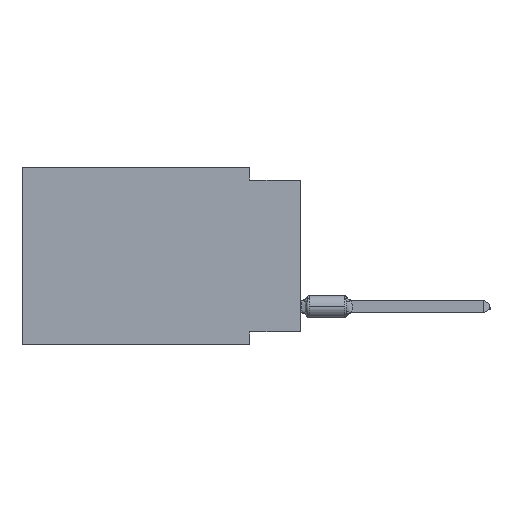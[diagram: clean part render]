
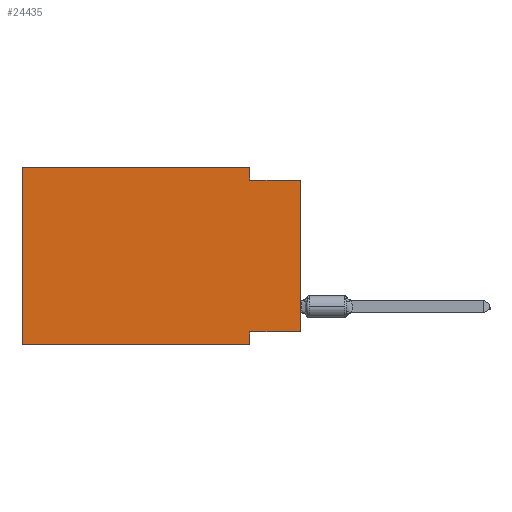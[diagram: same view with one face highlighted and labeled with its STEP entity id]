
A CAD part, left-side view. The second image highlights one B-rep face of the part: STEP entity #24435.
In plain terms, the highlighted planar face has unit normal (-1, 0, 0).
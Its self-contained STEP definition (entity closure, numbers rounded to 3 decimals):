
#930 = VECTOR ( 'NONE', #31908, 1000. ) ;
#1468 = ORIENTED_EDGE ( 'NONE', *, *, #15629, .T. ) ;
#1603 = VERTEX_POINT ( 'NONE', #9356 ) ;
#1657 = LINE ( 'NONE', #26154, #13521 ) ;
#1688 = LINE ( 'NONE', #13931, #12586 ) ;
#4065 = EDGE_CURVE ( 'NONE', #1603, #14126, #7188, .T. ) ;
#5180 = VECTOR ( 'NONE', #22248, 1000. ) ;
#5449 = AXIS2_PLACEMENT_3D ( 'NONE', #14521, #35636, #17737 ) ;
#5490 = ORIENTED_EDGE ( 'NONE', *, *, #20607, .F. ) ;
#6143 = DIRECTION ( 'NONE',  ( 0., -1., 0. ) ) ;
#7188 = LINE ( 'NONE', #19037, #5180 ) ;
#7659 = EDGE_CURVE ( 'NONE', #29925, #8269, #30034, .T. ) ;
#7812 = LINE ( 'NONE', #26083, #930 ) ;
#8269 = VERTEX_POINT ( 'NONE', #36052 ) ;
#8613 = EDGE_CURVE ( 'NONE', #14434, #14126, #1688, .T. ) ;
#9356 = CARTESIAN_POINT ( 'NONE',  ( 0., 2.54, -8.255 ) ) ;
#9601 = CARTESIAN_POINT ( 'NONE',  ( 0., 0., -8.255 ) ) ;
#11533 = CARTESIAN_POINT ( 'NONE',  ( 0., 13.97, 0. ) ) ;
#12391 = DIRECTION ( 'NONE',  ( 0., 0., -1. ) ) ;
#12416 = LINE ( 'NONE', #9601, #14799 ) ;
#12581 = DIRECTION ( 'NONE',  ( 0., 0., 1. ) ) ;
#12586 = VECTOR ( 'NONE', #23693, 1000. ) ;
#13521 = VECTOR ( 'NONE', #38407, 1000. ) ;
#13931 = CARTESIAN_POINT ( 'NONE',  ( 0., 13.97, -8.89 ) ) ;
#14126 = VERTEX_POINT ( 'NONE', #35458 ) ;
#14434 = VERTEX_POINT ( 'NONE', #31202 ) ;
#14521 = CARTESIAN_POINT ( 'NONE',  ( 0., 13.97, 0. ) ) ;
#14724 = VERTEX_POINT ( 'NONE', #27148 ) ;
#14799 = VECTOR ( 'NONE', #21839, 1000. ) ;
#15394 = LINE ( 'NONE', #27652, #16980 ) ;
#15629 = EDGE_CURVE ( 'NONE', #14724, #34569, #25978, .T. ) ;
#16320 = ORIENTED_EDGE ( 'NONE', *, *, #20735, .F. ) ;
#16980 = VECTOR ( 'NONE', #12391, 1000. ) ;
#17299 = ORIENTED_EDGE ( 'NONE', *, *, #7659, .F. ) ;
#17737 = DIRECTION ( 'NONE',  ( 0., 0., -1. ) ) ;
#19037 = CARTESIAN_POINT ( 'NONE',  ( 0., 2.54, -8.89 ) ) ;
#19344 = VERTEX_POINT ( 'NONE', #33121 ) ;
#20607 = EDGE_CURVE ( 'NONE', #14434, #29925, #1657, .T. ) ;
#20735 = EDGE_CURVE ( 'NONE', #14724, #1603, #12416, .T. ) ;
#20791 = CARTESIAN_POINT ( 'NONE',  ( 0., 13.97, 0. ) ) ;
#21015 = ORIENTED_EDGE ( 'NONE', *, *, #23897, .F. ) ;
#21839 = DIRECTION ( 'NONE',  ( 0., 1., 0. ) ) ;
#21958 = CARTESIAN_POINT ( 'NONE',  ( 0., 0., -0.635 ) ) ;
#22248 = DIRECTION ( 'NONE',  ( 0., 0., -1. ) ) ;
#23608 = EDGE_CURVE ( 'NONE', #19344, #34569, #7812, .T. ) ;
#23693 = DIRECTION ( 'NONE',  ( 0., -1., 0. ) ) ;
#23897 = EDGE_CURVE ( 'NONE', #8269, #19344, #15394, .T. ) ;
#24435 = ADVANCED_FACE ( 'NONE', ( #35431 ), #33189, .F. ) ;
#24822 = CARTESIAN_POINT ( 'NONE',  ( 0., 0., 0. ) ) ;
#25978 = LINE ( 'NONE', #24822, #30265 ) ;
#26083 = CARTESIAN_POINT ( 'NONE',  ( 0., 0., -0.635 ) ) ;
#26154 = CARTESIAN_POINT ( 'NONE',  ( 0., 13.97, 0. ) ) ;
#26357 = ORIENTED_EDGE ( 'NONE', *, *, #4065, .F. ) ;
#27148 = CARTESIAN_POINT ( 'NONE',  ( 0., 0., -8.255 ) ) ;
#27652 = CARTESIAN_POINT ( 'NONE',  ( 0., 2.54, 0. ) ) ;
#29925 = VERTEX_POINT ( 'NONE', #11533 ) ;
#30034 = LINE ( 'NONE', #20791, #36898 ) ;
#30265 = VECTOR ( 'NONE', #12581, 1000. ) ;
#31202 = CARTESIAN_POINT ( 'NONE',  ( 0., 13.97, -8.89 ) ) ;
#31908 = DIRECTION ( 'NONE',  ( 0., -1., 0. ) ) ;
#31910 = ORIENTED_EDGE ( 'NONE', *, *, #23608, .F. ) ;
#31990 = ORIENTED_EDGE ( 'NONE', *, *, #8613, .T. ) ;
#32360 = EDGE_LOOP ( 'NONE', ( #1468, #31910, #21015, #17299, #5490, #31990, #26357, #16320 ) ) ;
#33121 = CARTESIAN_POINT ( 'NONE',  ( 0., 2.54, -0.635 ) ) ;
#33189 = PLANE ( 'NONE',  #5449 ) ;
#34569 = VERTEX_POINT ( 'NONE', #21958 ) ;
#35431 = FACE_OUTER_BOUND ( 'NONE', #32360, .T. ) ;
#35458 = CARTESIAN_POINT ( 'NONE',  ( 0., 2.54, -8.89 ) ) ;
#35636 = DIRECTION ( 'NONE',  ( 1., 0., 0. ) ) ;
#36052 = CARTESIAN_POINT ( 'NONE',  ( 0., 2.54, 0. ) ) ;
#36898 = VECTOR ( 'NONE', #6143, 1000. ) ;
#38407 = DIRECTION ( 'NONE',  ( 0., 0., 1. ) ) ;
